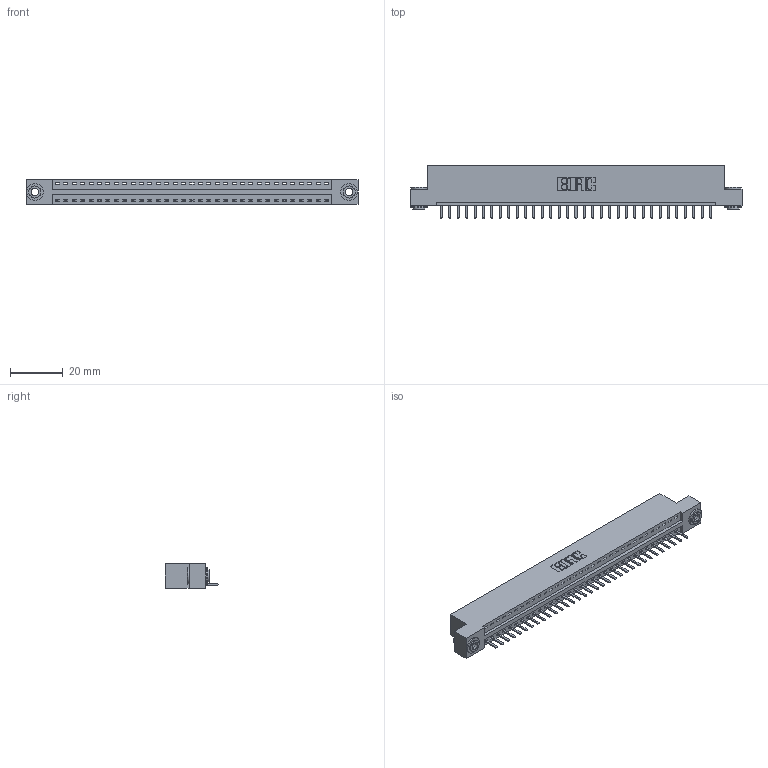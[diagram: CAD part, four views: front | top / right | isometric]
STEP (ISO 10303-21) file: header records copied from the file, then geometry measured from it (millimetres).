
FILE_DESCRIPTION (( 'STEP AP203' ), '1' );
FILE_NAME ('396-033-520-103.STEP', '2018-09-05T12:30:34', ( '' ), ( '' ), 'SwSTEP 2.0', 'SolidWorks 2016', '' );
FILE_SCHEMA (( 'CONFIG_CONTROL_DESIGN' ));
Length unit declared in the file: inch
Products named in the file (4): 345-250-002_345-250-002-102; 396-033-520-103; 346 Part_Flush Mounting Lugs - 0.156 Dia-TH; 345-292-001_345-293-120
Assembly tree (36 placements, depth 2):
  396-033-520-103
    346 Part_Flush Mounting Lugs - 0.156 Dia-TH
    345-292-001_345-293-120  x33
    345-250-002_345-250-002-102  x2
Bounding box: 125.35 x 20.02 x 9.4 mm (x, y, z)
Volume: 11861.1 mm3; surface area: 14630.1 mm2
Topology: 36 solids, 36 shells, 2206 faces, 6477 edges, 4226 vertices
Faces by surface type: plane 1472, cylinder 726, cone 8
Entity records: 22456 total; most frequent: CARTESIAN_POINT 3842, ORIENTED_EDGE 3790, DIRECTION 3419, EDGE_CURVE 1895, VECTOR 1603, LINE 1603, VERTEX_POINT 1258, AXIS2_PLACEMENT_3D 908
